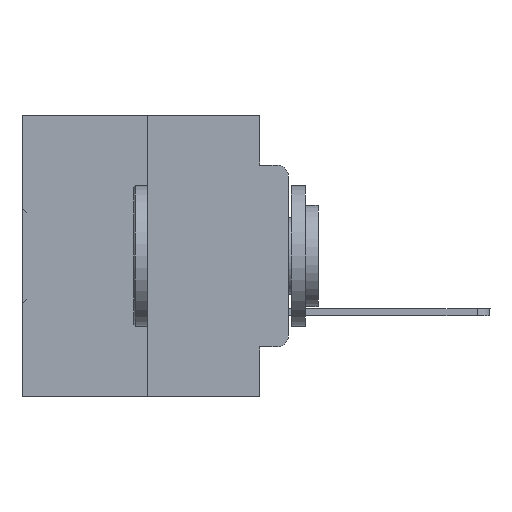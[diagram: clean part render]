
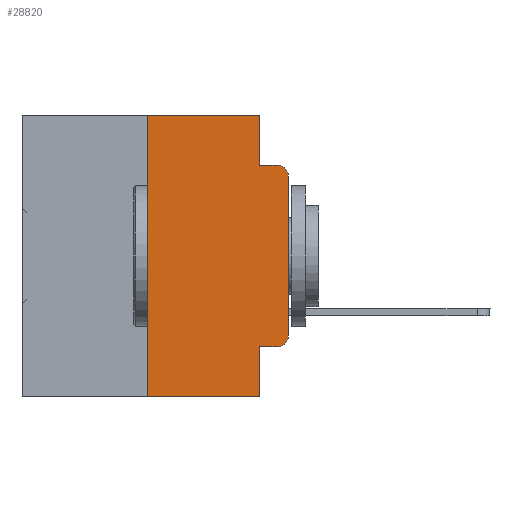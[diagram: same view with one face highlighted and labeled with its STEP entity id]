
A CAD part, left-side view. The second image highlights one B-rep face of the part: STEP entity #28820.
In plain terms, the highlighted planar face has unit normal (-1, 0, 0).
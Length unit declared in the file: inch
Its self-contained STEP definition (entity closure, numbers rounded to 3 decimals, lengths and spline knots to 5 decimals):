
#222 = AXIS2_PLACEMENT_3D ( 'NONE', #473, #13960, #24480 ) ;
#225 = CIRCLE ( 'NONE', #26709, 0.02 ) ;
#473 = CARTESIAN_POINT ( 'NONE',  ( 0., 0.473, 0. ) ) ;
#796 = VECTOR ( 'NONE', #26422, 39.37008 ) ;
#805 = PLANE ( 'NONE',  #222 ) ;
#907 = ORIENTED_EDGE ( 'NONE', *, *, #33668, .F. ) ;
#1491 = VERTEX_POINT ( 'NONE', #27740 ) ;
#1648 = VECTOR ( 'NONE', #16398, 39.37008 ) ;
#2776 = CARTESIAN_POINT ( 'NONE',  ( 0., 0.02, -0.3915 ) ) ;
#3083 = CARTESIAN_POINT ( 'NONE',  ( 0., 0.473, 0. ) ) ;
#3249 = CARTESIAN_POINT ( 'NONE',  ( 0., 0.02, -0.0885 ) ) ;
#4402 = CARTESIAN_POINT ( 'NONE',  ( 0., 0.051, -0.4115 ) ) ;
#4453 = VECTOR ( 'NONE', #15115, 39.37008 ) ;
#4533 = ORIENTED_EDGE ( 'NONE', *, *, #18461, .F. ) ;
#4657 = CARTESIAN_POINT ( 'NONE',  ( 0., 0.051, -0.0885 ) ) ;
#5109 = CARTESIAN_POINT ( 'NONE',  ( 0., 0.051, -0.4115 ) ) ;
#5484 = AXIS2_PLACEMENT_3D ( 'NONE', #19225, #19732, #30246 ) ;
#6022 = CARTESIAN_POINT ( 'NONE',  ( 0., 0.051, -0.5 ) ) ;
#6134 = CARTESIAN_POINT ( 'NONE',  ( 0., 0., -0.3915 ) ) ;
#8505 = EDGE_CURVE ( 'NONE', #21580, #11175, #225, .T. ) ;
#8818 = EDGE_CURVE ( 'NONE', #1491, #18623, #13468, .T. ) ;
#9015 = VERTEX_POINT ( 'NONE', #16741 ) ;
#9908 = DIRECTION ( 'NONE',  ( 0., -1., 0. ) ) ;
#9948 = LINE ( 'NONE', #4402, #4453 ) ;
#10823 = LINE ( 'NONE', #21341, #21942 ) ;
#11175 = VERTEX_POINT ( 'NONE', #6134 ) ;
#12073 = CARTESIAN_POINT ( 'NONE',  ( 0., 0.051, -0.0885 ) ) ;
#12988 = DIRECTION ( 'NONE',  ( -1., 0., 0. ) ) ;
#13468 = LINE ( 'NONE', #29337, #796 ) ;
#13960 = DIRECTION ( 'NONE',  ( 1., 0., 0. ) ) ;
#13981 = DIRECTION ( 'NONE',  ( 0., -1., 0. ) ) ;
#15115 = DIRECTION ( 'NONE',  ( 0., -1., 0. ) ) ;
#15205 = LINE ( 'NONE', #4657, #30709 ) ;
#16398 = DIRECTION ( 'NONE',  ( 0., 0., 1. ) ) ;
#16636 = ORIENTED_EDGE ( 'NONE', *, *, #17803, .T. ) ;
#16741 = CARTESIAN_POINT ( 'NONE',  ( 0., 0., -0.1085 ) ) ;
#17139 = EDGE_CURVE ( 'NONE', #22298, #33163, #29321, .T. ) ;
#17216 = VERTEX_POINT ( 'NONE', #3249 ) ;
#17803 = EDGE_CURVE ( 'NONE', #22298, #24695, #33495, .T. ) ;
#18461 = EDGE_CURVE ( 'NONE', #33163, #1491, #24504, .T. ) ;
#18623 = VERTEX_POINT ( 'NONE', #12073 ) ;
#19057 = VECTOR ( 'NONE', #13981, 39.37008 ) ;
#19225 = CARTESIAN_POINT ( 'NONE',  ( 0., 0.02, -0.1085 ) ) ;
#19249 = ORIENTED_EDGE ( 'NONE', *, *, #23882, .T. ) ;
#19276 = CARTESIAN_POINT ( 'NONE',  ( 0., 0.25, 0. ) ) ;
#19395 = DIRECTION ( 'NONE',  ( 0., -1., 0. ) ) ;
#19557 = LINE ( 'NONE', #27511, #27131 ) ;
#19732 = DIRECTION ( 'NONE',  ( -1., 0., 0. ) ) ;
#20382 = CIRCLE ( 'NONE', #5484, 0.02 ) ;
#21341 = CARTESIAN_POINT ( 'NONE',  ( 0., 0., 0. ) ) ;
#21517 = DIRECTION ( 'NONE',  ( 0., 0., 1. ) ) ;
#21546 = ORIENTED_EDGE ( 'NONE', *, *, #8818, .F. ) ;
#21580 = VERTEX_POINT ( 'NONE', #23971 ) ;
#21713 = FACE_OUTER_BOUND ( 'NONE', #33264, .T. ) ;
#21934 = VERTEX_POINT ( 'NONE', #5109 ) ;
#21942 = VECTOR ( 'NONE', #21517, 39.37008 ) ;
#21994 = EDGE_CURVE ( 'NONE', #11175, #9015, #10823, .T. ) ;
#22298 = VERTEX_POINT ( 'NONE', #31133 ) ;
#22511 = DIRECTION ( 'NONE',  ( 0., 0., -1. ) ) ;
#22838 = CARTESIAN_POINT ( 'NONE',  ( 0., 0.473, -0.5 ) ) ;
#23516 = DIRECTION ( 'NONE',  ( 0., 0., -1. ) ) ;
#23818 = CARTESIAN_POINT ( 'NONE',  ( 0., 0.25, 0. ) ) ;
#23882 = EDGE_CURVE ( 'NONE', #9015, #17216, #20382, .T. ) ;
#23971 = CARTESIAN_POINT ( 'NONE',  ( 0., 0.02, -0.4115 ) ) ;
#24480 = DIRECTION ( 'NONE',  ( 0., 0., -1. ) ) ;
#24504 = LINE ( 'NONE', #3083, #19057 ) ;
#24695 = VERTEX_POINT ( 'NONE', #6022 ) ;
#24921 = ORIENTED_EDGE ( 'NONE', *, *, #17139, .F. ) ;
#26212 = EDGE_CURVE ( 'NONE', #21934, #21580, #9948, .T. ) ;
#26346 = ORIENTED_EDGE ( 'NONE', *, *, #8505, .T. ) ;
#26422 = DIRECTION ( 'NONE',  ( 0., 0., -1. ) ) ;
#26709 = AXIS2_PLACEMENT_3D ( 'NONE', #2776, #12988, #23516 ) ;
#27131 = VECTOR ( 'NONE', #22511, 39.37008 ) ;
#27511 = CARTESIAN_POINT ( 'NONE',  ( 0., 0.051, 0. ) ) ;
#27730 = EDGE_CURVE ( 'NONE', #21934, #24695, #19557, .T. ) ;
#27740 = CARTESIAN_POINT ( 'NONE',  ( 0., 0.051, 0. ) ) ;
#28820 = ADVANCED_FACE ( 'NONE', ( #21713 ), #805, .F. ) ;
#29321 = LINE ( 'NONE', #23818, #1648 ) ;
#29337 = CARTESIAN_POINT ( 'NONE',  ( 0., 0.051, 0. ) ) ;
#30246 = DIRECTION ( 'NONE',  ( 0., 0., -1. ) ) ;
#30709 = VECTOR ( 'NONE', #19395, 39.37008 ) ;
#30995 = ORIENTED_EDGE ( 'NONE', *, *, #26212, .T. ) ;
#31133 = CARTESIAN_POINT ( 'NONE',  ( 0., 0.25, -0.5 ) ) ;
#32009 = ORIENTED_EDGE ( 'NONE', *, *, #21994, .T. ) ;
#32139 = ORIENTED_EDGE ( 'NONE', *, *, #27730, .F. ) ;
#33163 = VERTEX_POINT ( 'NONE', #19276 ) ;
#33264 = EDGE_LOOP ( 'NONE', ( #32009, #19249, #907, #21546, #4533, #24921, #16636, #32139, #30995, #26346 ) ) ;
#33328 = VECTOR ( 'NONE', #9908, 39.37008 ) ;
#33495 = LINE ( 'NONE', #22838, #33328 ) ;
#33668 = EDGE_CURVE ( 'NONE', #18623, #17216, #15205, .T. ) ;
